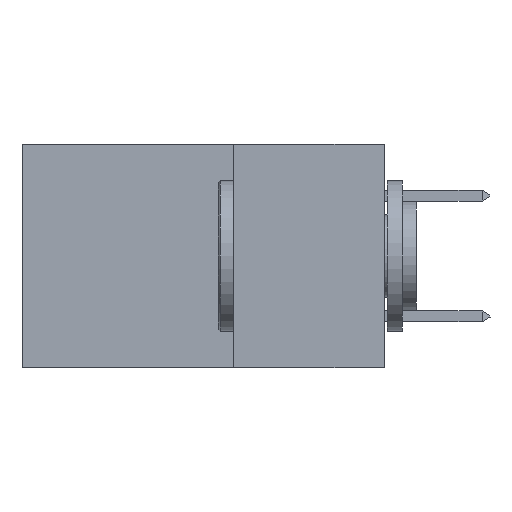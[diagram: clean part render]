
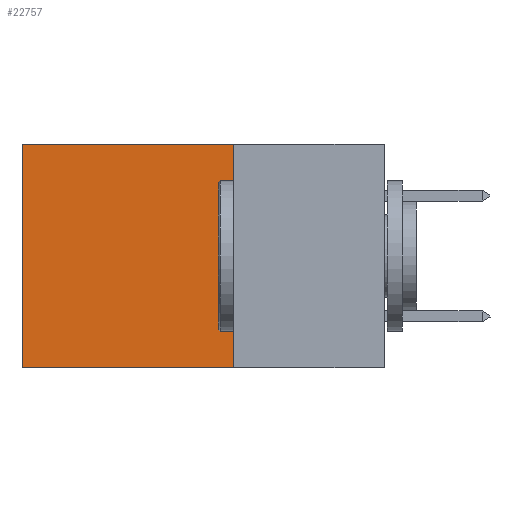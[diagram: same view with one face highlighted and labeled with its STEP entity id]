
A CAD part, left-side view. The second image highlights one B-rep face of the part: STEP entity #22757.
In plain terms, the highlighted planar face has unit normal (-1, 0, 0).
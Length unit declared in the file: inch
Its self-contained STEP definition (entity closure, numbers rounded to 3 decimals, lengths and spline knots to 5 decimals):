
#1118 = FACE_OUTER_BOUND ( 'NONE', #24477, .T. ) ;
#1400 = DIRECTION ( 'NONE',  ( 0., 0., -1. ) ) ;
#1541 = DIRECTION ( 'NONE',  ( 0., 0., -1. ) ) ;
#2352 = LINE ( 'NONE', #14218, #25143 ) ;
#2365 = LINE ( 'NONE', #13751, #25151 ) ;
#3057 = VERTEX_POINT ( 'NONE', #5117 ) ;
#3243 = LINE ( 'NONE', #21121, #13921 ) ;
#3812 = VERTEX_POINT ( 'NONE', #22045 ) ;
#5117 = CARTESIAN_POINT ( 'NONE',  ( 0.2875, 0.25, -0.37 ) ) ;
#9343 = ORIENTED_EDGE ( 'NONE', *, *, #13653, .F. ) ;
#9477 = DIRECTION ( 'NONE',  ( 0., 0., -1. ) ) ;
#10176 = DIRECTION ( 'NONE',  ( 0., 1., 0. ) ) ;
#10524 = ORIENTED_EDGE ( 'NONE', *, *, #28113, .F. ) ;
#10668 = PLANE ( 'NONE',  #21321 ) ;
#12102 = DIRECTION ( 'NONE',  ( 0., 1., 0. ) ) ;
#12582 = EDGE_CURVE ( 'NONE', #23184, #3812, #2365, .T. ) ;
#13003 = CARTESIAN_POINT ( 'NONE',  ( 0.2875, 0.25, 0. ) ) ;
#13621 = CARTESIAN_POINT ( 'NONE',  ( 0.2875, 0.25, 0. ) ) ;
#13653 = EDGE_CURVE ( 'NONE', #15023, #3057, #23558, .T. ) ;
#13751 = CARTESIAN_POINT ( 'NONE',  ( 0.2875, 0.6, 0. ) ) ;
#13921 = VECTOR ( 'NONE', #10176, 39.37008 ) ;
#14218 = CARTESIAN_POINT ( 'NONE',  ( 0.2875, 0.25, -0.37 ) ) ;
#15023 = VERTEX_POINT ( 'NONE', #13621 ) ;
#15080 = DIRECTION ( 'NONE',  ( 1., 0., 0. ) ) ;
#15404 = ORIENTED_EDGE ( 'NONE', *, *, #12582, .T. ) ;
#16517 = VECTOR ( 'NONE', #1541, 39.37008 ) ;
#21121 = CARTESIAN_POINT ( 'NONE',  ( 0.2875, 0.25, 0. ) ) ;
#21321 = AXIS2_PLACEMENT_3D ( 'NONE', #27736, #15080, #1400 ) ;
#22045 = CARTESIAN_POINT ( 'NONE',  ( 0.2875, 0.6, -0.37 ) ) ;
#22757 = ADVANCED_FACE ( 'NONE', ( #1118 ), #10668, .F. ) ;
#23184 = VERTEX_POINT ( 'NONE', #24849 ) ;
#23558 = LINE ( 'NONE', #13003, #16517 ) ;
#24477 = EDGE_LOOP ( 'NONE', ( #15404, #10524, #9343, #28318 ) ) ;
#24849 = CARTESIAN_POINT ( 'NONE',  ( 0.2875, 0.6, 0. ) ) ;
#25143 = VECTOR ( 'NONE', #12102, 39.37008 ) ;
#25151 = VECTOR ( 'NONE', #9477, 39.37008 ) ;
#25402 = EDGE_CURVE ( 'NONE', #15023, #23184, #3243, .T. ) ;
#27736 = CARTESIAN_POINT ( 'NONE',  ( 0.2875, 0.25, 0. ) ) ;
#28113 = EDGE_CURVE ( 'NONE', #3057, #3812, #2352, .T. ) ;
#28318 = ORIENTED_EDGE ( 'NONE', *, *, #25402, .T. ) ;
